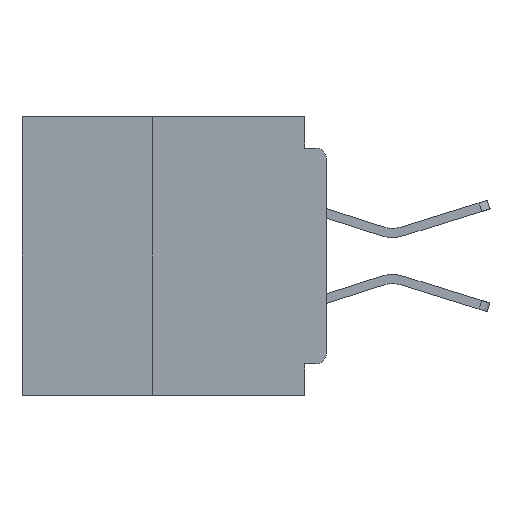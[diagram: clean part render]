
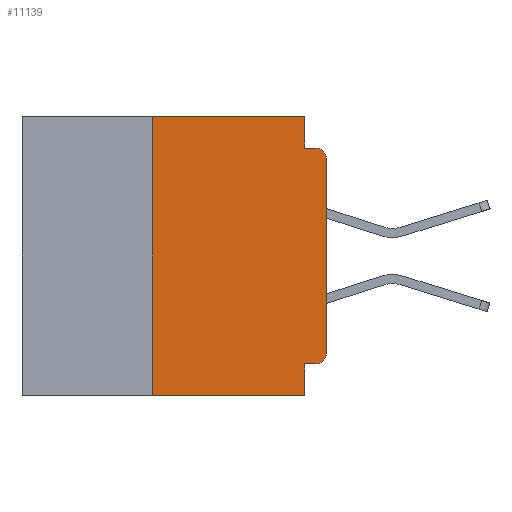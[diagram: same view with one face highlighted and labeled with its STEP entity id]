
A CAD part, left-side view. The second image highlights one B-rep face of the part: STEP entity #11139.
In plain terms, the highlighted planar face has unit normal (-1, 0, 0).
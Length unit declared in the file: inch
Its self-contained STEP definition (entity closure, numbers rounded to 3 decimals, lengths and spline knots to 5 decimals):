
#521 = CARTESIAN_POINT ( 'NONE',  ( 0., 0.031, -0.4 ) ) ;
#1466 = PLANE ( 'NONE',  #41827 ) ;
#2333 = CARTESIAN_POINT ( 'NONE',  ( 0., 0., -0.045 ) ) ;
#3286 = FACE_OUTER_BOUND ( 'NONE', #62310, .T. ) ;
#3405 = VERTEX_POINT ( 'NONE', #21527 ) ;
#5308 = CARTESIAN_POINT ( 'NONE',  ( 0., 0.031, -0.4 ) ) ;
#6523 = DIRECTION ( 'NONE',  ( 0., 0., -1. ) ) ;
#7893 = CARTESIAN_POINT ( 'NONE',  ( 0., 0.015, -0.34 ) ) ;
#8751 = VECTOR ( 'NONE', #39073, 39.37008 ) ;
#9003 = EDGE_CURVE ( 'NONE', #3405, #47254, #28805, .T. ) ;
#9106 = CARTESIAN_POINT ( 'NONE',  ( 0., 0.437, -0.4 ) ) ;
#10331 = LINE ( 'NONE', #34016, #8751 ) ;
#11035 = VECTOR ( 'NONE', #45725, 39.37008 ) ;
#11139 = ADVANCED_FACE ( 'NONE', ( #3286 ), #1466, .F. ) ;
#11924 = LINE ( 'NONE', #9106, #35599 ) ;
#12483 = VERTEX_POINT ( 'NONE', #27797 ) ;
#12676 = VERTEX_POINT ( 'NONE', #33929 ) ;
#12941 = DIRECTION ( 'NONE',  ( 0., 0., -1. ) ) ;
#13022 = CARTESIAN_POINT ( 'NONE',  ( 0., 0., 0. ) ) ;
#13875 = CARTESIAN_POINT ( 'NONE',  ( 0., 0., -0.34 ) ) ;
#14219 = LINE ( 'NONE', #5308, #11035 ) ;
#15253 = DIRECTION ( 'NONE',  ( 0., 0., -1. ) ) ;
#16179 = ORIENTED_EDGE ( 'NONE', *, *, #24285, .F. ) ;
#16661 = LINE ( 'NONE', #47502, #55137 ) ;
#16924 = EDGE_CURVE ( 'NONE', #53629, #3405, #51547, .T. ) ;
#17276 = VERTEX_POINT ( 'NONE', #60618 ) ;
#17540 = CARTESIAN_POINT ( 'NONE',  ( 0., 0.25, 0. ) ) ;
#18517 = AXIS2_PLACEMENT_3D ( 'NONE', #7893, #43053, #12941 ) ;
#20547 = DIRECTION ( 'NONE',  ( -1., 0., 0. ) ) ;
#21527 = CARTESIAN_POINT ( 'NONE',  ( 0., 0., -0.06 ) ) ;
#22554 = VECTOR ( 'NONE', #15253, 39.37008 ) ;
#23686 = CARTESIAN_POINT ( 'NONE',  ( 0., 0.031, 0. ) ) ;
#24285 = EDGE_CURVE ( 'NONE', #12483, #31931, #14219, .T. ) ;
#27429 = DIRECTION ( 'NONE',  ( 0., -1., 0. ) ) ;
#27487 = DIRECTION ( 'NONE',  ( 0., -1., 0. ) ) ;
#27559 = AXIS2_PLACEMENT_3D ( 'NONE', #50587, #20547, #55618 ) ;
#27797 = CARTESIAN_POINT ( 'NONE',  ( 0., 0.031, -0.355 ) ) ;
#28061 = VECTOR ( 'NONE', #27487, 39.37008 ) ;
#28641 = ORIENTED_EDGE ( 'NONE', *, *, #30091, .F. ) ;
#28805 = CIRCLE ( 'NONE', #27559, 0.015 ) ;
#29657 = LINE ( 'NONE', #62339, #28061 ) ;
#30091 = EDGE_CURVE ( 'NONE', #60692, #12676, #49227, .T. ) ;
#30914 = EDGE_CURVE ( 'NONE', #31571, #60692, #29657, .T. ) ;
#31571 = VERTEX_POINT ( 'NONE', #17540 ) ;
#31931 = VERTEX_POINT ( 'NONE', #521 ) ;
#33929 = CARTESIAN_POINT ( 'NONE',  ( 0., 0.031, -0.045 ) ) ;
#34016 = CARTESIAN_POINT ( 'NONE',  ( 0., 0.25, -0.4 ) ) ;
#34191 = DIRECTION ( 'NONE',  ( 0., -1., 0. ) ) ;
#34729 = ORIENTED_EDGE ( 'NONE', *, *, #9003, .T. ) ;
#35599 = VECTOR ( 'NONE', #34191, 39.37008 ) ;
#35805 = EDGE_CURVE ( 'NONE', #17276, #31571, #10331, .T. ) ;
#35865 = VERTEX_POINT ( 'NONE', #44523 ) ;
#36712 = DIRECTION ( 'NONE',  ( 1., 0., 0. ) ) ;
#38459 = ORIENTED_EDGE ( 'NONE', *, *, #30914, .F. ) ;
#38876 = CIRCLE ( 'NONE', #18517, 0.015 ) ;
#39073 = DIRECTION ( 'NONE',  ( 0., 0., 1. ) ) ;
#39513 = ORIENTED_EDGE ( 'NONE', *, *, #35805, .F. ) ;
#39829 = VECTOR ( 'NONE', #48154, 39.37008 ) ;
#41827 = AXIS2_PLACEMENT_3D ( 'NONE', #61652, #36712, #6523 ) ;
#42472 = DIRECTION ( 'NONE',  ( 0., 1., 0. ) ) ;
#43053 = DIRECTION ( 'NONE',  ( -1., 0., 0. ) ) ;
#43221 = EDGE_CURVE ( 'NONE', #35865, #53629, #38876, .T. ) ;
#43429 = CARTESIAN_POINT ( 'NONE',  ( 0., 0.015, -0.045 ) ) ;
#44192 = ORIENTED_EDGE ( 'NONE', *, *, #61953, .T. ) ;
#44446 = EDGE_CURVE ( 'NONE', #35865, #12483, #16661, .T. ) ;
#44523 = CARTESIAN_POINT ( 'NONE',  ( 0., 0.015, -0.355 ) ) ;
#45656 = EDGE_CURVE ( 'NONE', #12676, #47254, #62791, .T. ) ;
#45725 = DIRECTION ( 'NONE',  ( 0., 0., -1. ) ) ;
#46206 = ORIENTED_EDGE ( 'NONE', *, *, #16924, .T. ) ;
#47254 = VERTEX_POINT ( 'NONE', #43429 ) ;
#47502 = CARTESIAN_POINT ( 'NONE',  ( 0., 0., -0.355 ) ) ;
#48154 = DIRECTION ( 'NONE',  ( 0., 0., 1. ) ) ;
#49227 = LINE ( 'NONE', #50167, #22554 ) ;
#49449 = VECTOR ( 'NONE', #27429, 39.37008 ) ;
#50167 = CARTESIAN_POINT ( 'NONE',  ( 0., 0.031, 0. ) ) ;
#50587 = CARTESIAN_POINT ( 'NONE',  ( 0., 0.015, -0.06 ) ) ;
#51547 = LINE ( 'NONE', #13022, #39829 ) ;
#53629 = VERTEX_POINT ( 'NONE', #13875 ) ;
#55137 = VECTOR ( 'NONE', #42472, 39.37008 ) ;
#55618 = DIRECTION ( 'NONE',  ( 0., 0., -1. ) ) ;
#57582 = ORIENTED_EDGE ( 'NONE', *, *, #44446, .F. ) ;
#59870 = ORIENTED_EDGE ( 'NONE', *, *, #43221, .T. ) ;
#60572 = ORIENTED_EDGE ( 'NONE', *, *, #45656, .F. ) ;
#60618 = CARTESIAN_POINT ( 'NONE',  ( 0., 0.25, -0.4 ) ) ;
#60692 = VERTEX_POINT ( 'NONE', #23686 ) ;
#61652 = CARTESIAN_POINT ( 'NONE',  ( 0., 0.437, 0. ) ) ;
#61953 = EDGE_CURVE ( 'NONE', #17276, #31931, #11924, .T. ) ;
#62310 = EDGE_LOOP ( 'NONE', ( #46206, #34729, #60572, #28641, #38459, #39513, #44192, #16179, #57582, #59870 ) ) ;
#62339 = CARTESIAN_POINT ( 'NONE',  ( 0., 0.437, 0. ) ) ;
#62791 = LINE ( 'NONE', #2333, #49449 ) ;
